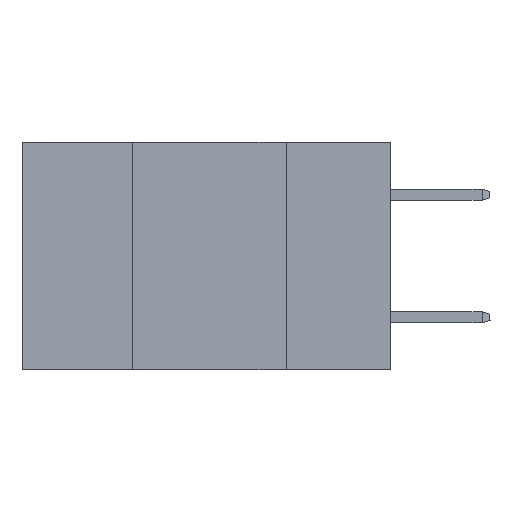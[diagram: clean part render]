
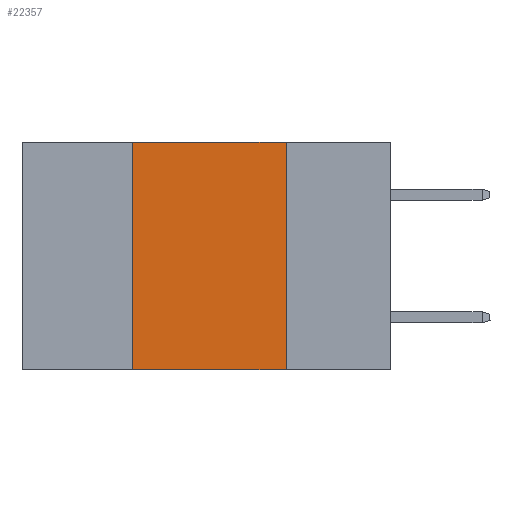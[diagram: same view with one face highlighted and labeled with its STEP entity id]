
A CAD part, left-side view. The second image highlights one B-rep face of the part: STEP entity #22357.
In plain terms, the highlighted planar face has unit normal (-1, 0, 0).
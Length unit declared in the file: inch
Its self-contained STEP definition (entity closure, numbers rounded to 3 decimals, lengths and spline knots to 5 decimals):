
#1714 = EDGE_CURVE ( 'NONE', #20142, #26532, #7290, .T. ) ;
#2130 = CARTESIAN_POINT ( 'NONE',  ( 0., 0.17, -0.37 ) ) ;
#3189 = AXIS2_PLACEMENT_3D ( 'NONE', #19861, #21672, #16252 ) ;
#3643 = EDGE_CURVE ( 'NONE', #33747, #26532, #37770, .T. ) ;
#3955 = LINE ( 'NONE', #7416, #32996 ) ;
#4571 = CARTESIAN_POINT ( 'NONE',  ( 0., 0.17, 0. ) ) ;
#7290 = LINE ( 'NONE', #4571, #15867 ) ;
#7416 = CARTESIAN_POINT ( 'NONE',  ( 0., 0.42, 0. ) ) ;
#7978 = ORIENTED_EDGE ( 'NONE', *, *, #3643, .T. ) ;
#8064 = PLANE ( 'NONE',  #3189 ) ;
#9434 = ORIENTED_EDGE ( 'NONE', *, *, #26706, .F. ) ;
#13797 = VERTEX_POINT ( 'NONE', #34321 ) ;
#15754 = DIRECTION ( 'NONE',  ( 0., 0., 1. ) ) ;
#15867 = VECTOR ( 'NONE', #19653, 39.37008 ) ;
#16252 = DIRECTION ( 'NONE',  ( 0., 0., -1. ) ) ;
#16790 = ORIENTED_EDGE ( 'NONE', *, *, #25874, .F. ) ;
#19653 = DIRECTION ( 'NONE',  ( 0., 0., -1. ) ) ;
#19839 = DIRECTION ( 'NONE',  ( 0., -1., 0. ) ) ;
#19861 = CARTESIAN_POINT ( 'NONE',  ( 0., 0.6, 0. ) ) ;
#20142 = VERTEX_POINT ( 'NONE', #36239 ) ;
#20829 = CARTESIAN_POINT ( 'NONE',  ( 0., 0.6, 0. ) ) ;
#21672 = DIRECTION ( 'NONE',  ( 1., 0., 0. ) ) ;
#22239 = FACE_OUTER_BOUND ( 'NONE', #30987, .T. ) ;
#22357 = ADVANCED_FACE ( 'NONE', ( #22239 ), #8064, .F. ) ;
#24498 = DIRECTION ( 'NONE',  ( 0., -1., 0. ) ) ;
#24943 = VECTOR ( 'NONE', #24498, 39.37008 ) ;
#25874 = EDGE_CURVE ( 'NONE', #33747, #13797, #3955, .T. ) ;
#26532 = VERTEX_POINT ( 'NONE', #2130 ) ;
#26706 = EDGE_CURVE ( 'NONE', #13797, #20142, #26828, .T. ) ;
#26828 = LINE ( 'NONE', #20829, #24943 ) ;
#30368 = VECTOR ( 'NONE', #19839, 39.37008 ) ;
#30987 = EDGE_LOOP ( 'NONE', ( #36237, #9434, #16790, #7978 ) ) ;
#32578 = CARTESIAN_POINT ( 'NONE',  ( 0., 0.42, -0.37 ) ) ;
#32996 = VECTOR ( 'NONE', #15754, 39.37008 ) ;
#33747 = VERTEX_POINT ( 'NONE', #32578 ) ;
#34321 = CARTESIAN_POINT ( 'NONE',  ( 0., 0.42, 0. ) ) ;
#34898 = CARTESIAN_POINT ( 'NONE',  ( 0., 0.6, -0.37 ) ) ;
#36237 = ORIENTED_EDGE ( 'NONE', *, *, #1714, .F. ) ;
#36239 = CARTESIAN_POINT ( 'NONE',  ( 0., 0.17, 0. ) ) ;
#37770 = LINE ( 'NONE', #34898, #30368 ) ;
